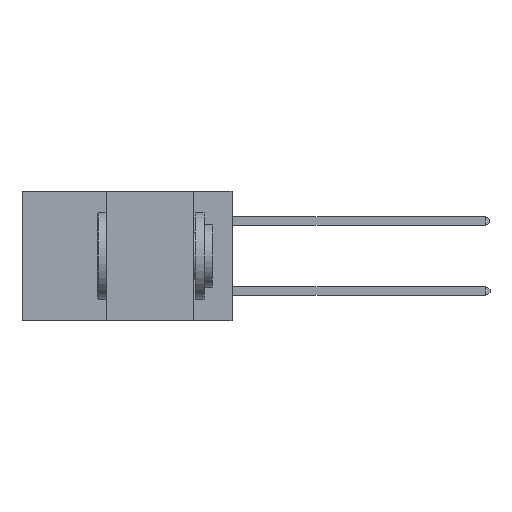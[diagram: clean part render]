
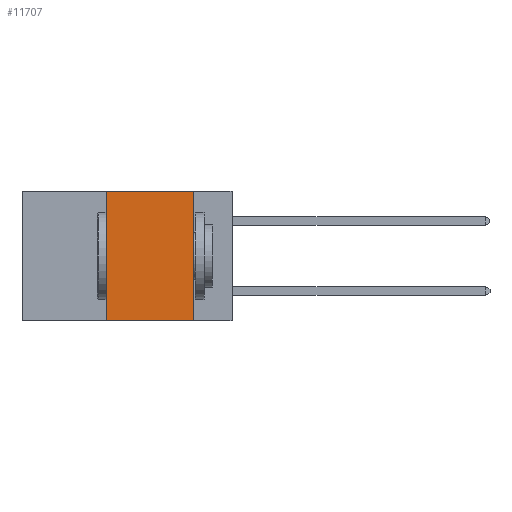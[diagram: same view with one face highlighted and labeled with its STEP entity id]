
A CAD part, left-side view. The second image highlights one B-rep face of the part: STEP entity #11707.
In plain terms, the highlighted planar face has unit normal (-1, 0, 0).
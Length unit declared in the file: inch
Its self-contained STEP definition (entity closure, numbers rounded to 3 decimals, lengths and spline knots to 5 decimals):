
#1224 = FACE_OUTER_BOUND ( 'NONE', #19532, .T. ) ;
#1235 = LINE ( 'NONE', #14924, #18603 ) ;
#1324 = CARTESIAN_POINT ( 'NONE',  ( 0., 0.6, 0. ) ) ;
#2907 = DIRECTION ( 'NONE',  ( 0., 0., 1. ) ) ;
#3197 = DIRECTION ( 'NONE',  ( 0., 0., -1. ) ) ;
#3226 = ORIENTED_EDGE ( 'NONE', *, *, #12929, .T. ) ;
#3267 = DIRECTION ( 'NONE',  ( 0., 0., -1. ) ) ;
#3516 = LINE ( 'NONE', #15282, #12611 ) ;
#3547 = VERTEX_POINT ( 'NONE', #7945 ) ;
#3762 = EDGE_CURVE ( 'NONE', #3547, #12921, #3516, .T. ) ;
#4179 = ORIENTED_EDGE ( 'NONE', *, *, #20318, .F. ) ;
#4223 = ORIENTED_EDGE ( 'NONE', *, *, #9215, .F. ) ;
#4395 = VECTOR ( 'NONE', #8521, 39.37008 ) ;
#6756 = CARTESIAN_POINT ( 'NONE',  ( 0., 0.6, -0.37 ) ) ;
#7402 = VERTEX_POINT ( 'NONE', #13223 ) ;
#7945 = CARTESIAN_POINT ( 'NONE',  ( 0., 0.11, 0. ) ) ;
#8115 = VECTOR ( 'NONE', #8482, 39.37008 ) ;
#8303 = PLANE ( 'NONE',  #10858 ) ;
#8482 = DIRECTION ( 'NONE',  ( 0., -1., 0. ) ) ;
#8500 = LINE ( 'NONE', #20513, #4395 ) ;
#8521 = DIRECTION ( 'NONE',  ( 0., -1., 0. ) ) ;
#8529 = CARTESIAN_POINT ( 'NONE',  ( 0., 0.36, -0.37 ) ) ;
#8580 = ORIENTED_EDGE ( 'NONE', *, *, #3762, .F. ) ;
#9215 = EDGE_CURVE ( 'NONE', #7402, #3547, #8500, .T. ) ;
#10858 = AXIS2_PLACEMENT_3D ( 'NONE', #1324, #13472, #3197 ) ;
#11707 = ADVANCED_FACE ( 'NONE', ( #1224 ), #8303, .F. ) ;
#11746 = VERTEX_POINT ( 'NONE', #8529 ) ;
#12584 = LINE ( 'NONE', #6756, #8115 ) ;
#12611 = VECTOR ( 'NONE', #3267, 39.37008 ) ;
#12921 = VERTEX_POINT ( 'NONE', #16925 ) ;
#12929 = EDGE_CURVE ( 'NONE', #11746, #12921, #12584, .T. ) ;
#13223 = CARTESIAN_POINT ( 'NONE',  ( 0., 0.36, 0. ) ) ;
#13472 = DIRECTION ( 'NONE',  ( 1., 0., 0. ) ) ;
#14924 = CARTESIAN_POINT ( 'NONE',  ( 0., 0.36, 0. ) ) ;
#15282 = CARTESIAN_POINT ( 'NONE',  ( 0., 0.11, 0. ) ) ;
#16925 = CARTESIAN_POINT ( 'NONE',  ( 0., 0.11, -0.37 ) ) ;
#18603 = VECTOR ( 'NONE', #2907, 39.37008 ) ;
#19532 = EDGE_LOOP ( 'NONE', ( #8580, #4223, #4179, #3226 ) ) ;
#20318 = EDGE_CURVE ( 'NONE', #11746, #7402, #1235, .T. ) ;
#20513 = CARTESIAN_POINT ( 'NONE',  ( 0., 0.6, 0. ) ) ;
